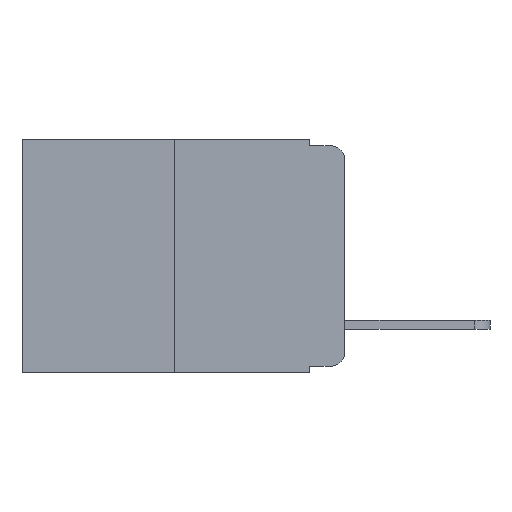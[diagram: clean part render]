
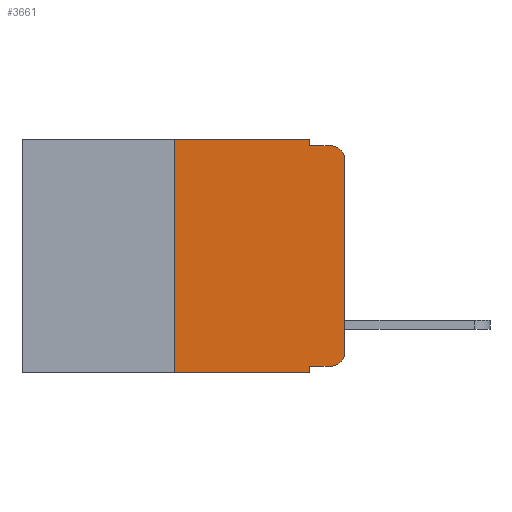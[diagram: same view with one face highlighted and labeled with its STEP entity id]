
A CAD part, left-side view. The second image highlights one B-rep face of the part: STEP entity #3661.
In plain terms, the highlighted planar face has unit normal (-1, 0, 0).
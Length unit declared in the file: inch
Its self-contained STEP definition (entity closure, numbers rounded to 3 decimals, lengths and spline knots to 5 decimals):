
#32 = ORIENTED_EDGE ( 'NONE', *, *, #6465, .F. ) ;
#87 = ORIENTED_EDGE ( 'NONE', *, *, #1693, .T. ) ;
#167 = ORIENTED_EDGE ( 'NONE', *, *, #9369, .T. ) ;
#306 = LINE ( 'NONE', #10653, #3169 ) ;
#764 = DIRECTION ( 'NONE',  ( 0., 0., -1. ) ) ;
#874 = CARTESIAN_POINT ( 'NONE',  ( 0., 0.051, -0.01 ) ) ;
#1032 = CARTESIAN_POINT ( 'NONE',  ( 0., 0., -0.03 ) ) ;
#1087 = EDGE_LOOP ( 'NONE', ( #5159, #5367, #11535, #6696, #9206, #10863, #11043, #32, #87, #167 ) ) ;
#1693 = EDGE_CURVE ( 'NONE', #7774, #9505, #2380, .T. ) ;
#1821 = CARTESIAN_POINT ( 'NONE',  ( 0., 0.473, 0. ) ) ;
#2133 = DIRECTION ( 'NONE',  ( -1., 0., 0. ) ) ;
#2249 = CARTESIAN_POINT ( 'NONE',  ( 0., 0., -0.313 ) ) ;
#2366 = VECTOR ( 'NONE', #8072, 39.37008 ) ;
#2380 = LINE ( 'NONE', #6174, #2366 ) ;
#2477 = FACE_OUTER_BOUND ( 'NONE', #1087, .T. ) ;
#3149 = VERTEX_POINT ( 'NONE', #11210 ) ;
#3169 = VECTOR ( 'NONE', #11470, 39.37008 ) ;
#3181 = LINE ( 'NONE', #874, #7036 ) ;
#3661 = ADVANCED_FACE ( 'NONE', ( #2477 ), #10171, .F. ) ;
#3798 = CARTESIAN_POINT ( 'NONE',  ( 0., 0.051, -0.01 ) ) ;
#3815 = AXIS2_PLACEMENT_3D ( 'NONE', #5986, #11928, #10382 ) ;
#3928 = DIRECTION ( 'NONE',  ( 0., -1., 0. ) ) ;
#4381 = VERTEX_POINT ( 'NONE', #5487 ) ;
#4510 = CIRCLE ( 'NONE', #9736, 0.02 ) ;
#4594 = EDGE_CURVE ( 'NONE', #6492, #4381, #6205, .T. ) ;
#4661 = VERTEX_POINT ( 'NONE', #2249 ) ;
#4949 = VECTOR ( 'NONE', #12005, 39.37008 ) ;
#5159 = ORIENTED_EDGE ( 'NONE', *, *, #5630, .T. ) ;
#5367 = ORIENTED_EDGE ( 'NONE', *, *, #5817, .T. ) ;
#5487 = CARTESIAN_POINT ( 'NONE',  ( 0., 0.051, 0. ) ) ;
#5630 = EDGE_CURVE ( 'NONE', #4661, #11384, #10444, .T. ) ;
#5817 = EDGE_CURVE ( 'NONE', #11384, #6412, #10869, .T. ) ;
#5946 = EDGE_CURVE ( 'NONE', #9219, #6412, #3181, .T. ) ;
#5986 = CARTESIAN_POINT ( 'NONE',  ( 0., 0.473, 0. ) ) ;
#6072 = VECTOR ( 'NONE', #3928, 39.37008 ) ;
#6174 = CARTESIAN_POINT ( 'NONE',  ( 0., 0.051, -0.333 ) ) ;
#6178 = DIRECTION ( 'NONE',  ( -1., 0., 0. ) ) ;
#6194 = CARTESIAN_POINT ( 'NONE',  ( 0., 0.02, -0.313 ) ) ;
#6205 = LINE ( 'NONE', #1821, #6072 ) ;
#6274 = EDGE_CURVE ( 'NONE', #4381, #9219, #7382, .T. ) ;
#6412 = VERTEX_POINT ( 'NONE', #10669 ) ;
#6419 = EDGE_CURVE ( 'NONE', #3149, #6492, #306, .T. ) ;
#6465 = EDGE_CURVE ( 'NONE', #7774, #6913, #12520, .T. ) ;
#6492 = VERTEX_POINT ( 'NONE', #12140 ) ;
#6557 = CARTESIAN_POINT ( 'NONE',  ( 0., 0.051, -0.333 ) ) ;
#6588 = DIRECTION ( 'NONE',  ( 0., 0., -1. ) ) ;
#6696 = ORIENTED_EDGE ( 'NONE', *, *, #6274, .F. ) ;
#6913 = VERTEX_POINT ( 'NONE', #8635 ) ;
#7036 = VECTOR ( 'NONE', #7348, 39.37008 ) ;
#7348 = DIRECTION ( 'NONE',  ( 0., -1., 0. ) ) ;
#7382 = LINE ( 'NONE', #12163, #4949 ) ;
#7774 = VERTEX_POINT ( 'NONE', #6557 ) ;
#8072 = DIRECTION ( 'NONE',  ( 0., -1., 0. ) ) ;
#8635 = CARTESIAN_POINT ( 'NONE',  ( 0., 0.051, -0.343 ) ) ;
#9206 = ORIENTED_EDGE ( 'NONE', *, *, #4594, .F. ) ;
#9219 = VERTEX_POINT ( 'NONE', #3798 ) ;
#9369 = EDGE_CURVE ( 'NONE', #9505, #4661, #4510, .T. ) ;
#9505 = VERTEX_POINT ( 'NONE', #11918 ) ;
#9532 = CARTESIAN_POINT ( 'NONE',  ( 0., 0., 0. ) ) ;
#9619 = CARTESIAN_POINT ( 'NONE',  ( 0., 0.02, -0.03 ) ) ;
#9736 = AXIS2_PLACEMENT_3D ( 'NONE', #6194, #6178, #6588 ) ;
#10002 = DIRECTION ( 'NONE',  ( 0., -1., 0. ) ) ;
#10059 = CARTESIAN_POINT ( 'NONE',  ( 0., 0.473, -0.343 ) ) ;
#10171 = PLANE ( 'NONE',  #3815 ) ;
#10382 = DIRECTION ( 'NONE',  ( 0., 0., -1. ) ) ;
#10420 = VECTOR ( 'NONE', #764, 39.37008 ) ;
#10444 = LINE ( 'NONE', #9532, #12332 ) ;
#10451 = AXIS2_PLACEMENT_3D ( 'NONE', #9619, #2133, #10728 ) ;
#10653 = CARTESIAN_POINT ( 'NONE',  ( 0., 0.25, 0. ) ) ;
#10669 = CARTESIAN_POINT ( 'NONE',  ( 0., 0.02, -0.01 ) ) ;
#10728 = DIRECTION ( 'NONE',  ( 0., 0., -1. ) ) ;
#10863 = ORIENTED_EDGE ( 'NONE', *, *, #6419, .F. ) ;
#10869 = CIRCLE ( 'NONE', #10451, 0.02 ) ;
#11043 = ORIENTED_EDGE ( 'NONE', *, *, #11747, .T. ) ;
#11210 = CARTESIAN_POINT ( 'NONE',  ( 0., 0.25, -0.343 ) ) ;
#11384 = VERTEX_POINT ( 'NONE', #1032 ) ;
#11470 = DIRECTION ( 'NONE',  ( 0., 0., 1. ) ) ;
#11535 = ORIENTED_EDGE ( 'NONE', *, *, #5946, .F. ) ;
#11747 = EDGE_CURVE ( 'NONE', #3149, #6913, #12238, .T. ) ;
#11793 = CARTESIAN_POINT ( 'NONE',  ( 0., 0.051, 0. ) ) ;
#11918 = CARTESIAN_POINT ( 'NONE',  ( 0., 0.02, -0.333 ) ) ;
#11928 = DIRECTION ( 'NONE',  ( 1., 0., 0. ) ) ;
#12005 = DIRECTION ( 'NONE',  ( 0., 0., -1. ) ) ;
#12009 = VECTOR ( 'NONE', #10002, 39.37008 ) ;
#12140 = CARTESIAN_POINT ( 'NONE',  ( 0., 0.25, 0. ) ) ;
#12163 = CARTESIAN_POINT ( 'NONE',  ( 0., 0.051, 0. ) ) ;
#12238 = LINE ( 'NONE', #10059, #12009 ) ;
#12332 = VECTOR ( 'NONE', #12485, 39.37008 ) ;
#12485 = DIRECTION ( 'NONE',  ( 0., 0., 1. ) ) ;
#12520 = LINE ( 'NONE', #11793, #10420 ) ;
